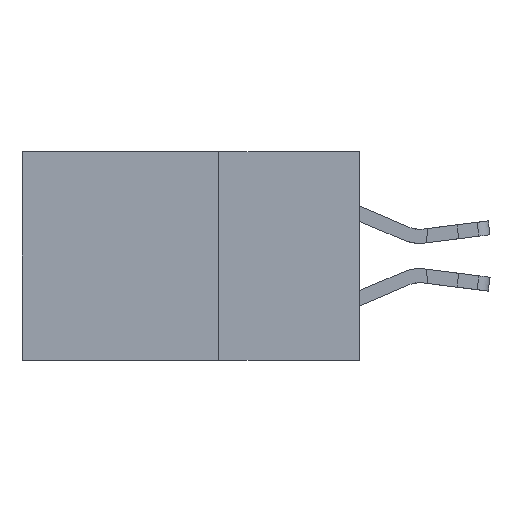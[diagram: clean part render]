
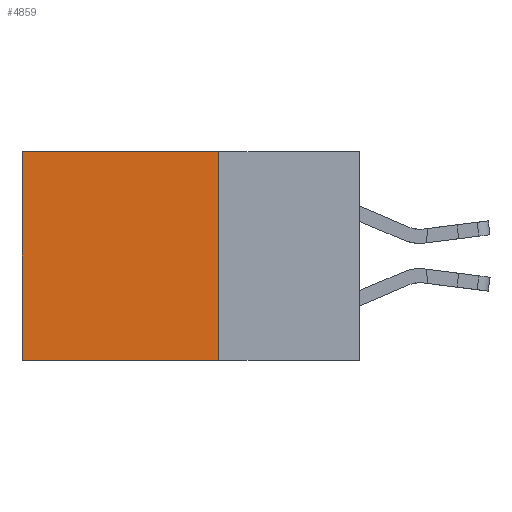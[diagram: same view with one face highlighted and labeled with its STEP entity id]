
A CAD part, left-side view. The second image highlights one B-rep face of the part: STEP entity #4859.
In plain terms, the highlighted planar face has unit normal (-1, 0, 0).
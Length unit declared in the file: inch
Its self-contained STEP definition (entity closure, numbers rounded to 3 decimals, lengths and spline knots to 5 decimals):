
#302 = EDGE_CURVE ( 'NONE', #24637, #29451, #16012, .T. ) ;
#420 = ORIENTED_EDGE ( 'NONE', *, *, #27359, .T. ) ;
#3857 = ORIENTED_EDGE ( 'NONE', *, *, #10901, .T. ) ;
#4203 = VECTOR ( 'NONE', #13015, 39.37008 ) ;
#4370 = DIRECTION ( 'NONE',  ( 0., 0., -1. ) ) ;
#4859 = ADVANCED_FACE ( 'NONE', ( #28854 ), #28910, .F. ) ;
#6079 = ORIENTED_EDGE ( 'NONE', *, *, #302, .F. ) ;
#6340 = ORIENTED_EDGE ( 'NONE', *, *, #11424, .F. ) ;
#8848 = CARTESIAN_POINT ( 'NONE',  ( 0.2875, 0.6, 0. ) ) ;
#9048 = LINE ( 'NONE', #17843, #19041 ) ;
#10865 = DIRECTION ( 'NONE',  ( 1., 0., 0. ) ) ;
#10901 = EDGE_CURVE ( 'NONE', #28396, #12480, #9048, .T. ) ;
#11424 = EDGE_CURVE ( 'NONE', #29451, #12480, #16415, .T. ) ;
#12384 = DIRECTION ( 'NONE',  ( 0., 0., -1. ) ) ;
#12480 = VERTEX_POINT ( 'NONE', #19694 ) ;
#13015 = DIRECTION ( 'NONE',  ( 0., 1., 0. ) ) ;
#13326 = DIRECTION ( 'NONE',  ( 0., 0., -1. ) ) ;
#13767 = CARTESIAN_POINT ( 'NONE',  ( 0.2875, 0.25, 0. ) ) ;
#14793 = CARTESIAN_POINT ( 'NONE',  ( 0.2875, 0.25, 0. ) ) ;
#16012 = LINE ( 'NONE', #16991, #21148 ) ;
#16415 = LINE ( 'NONE', #26955, #4203 ) ;
#16435 = DIRECTION ( 'NONE',  ( 0., 1., 0. ) ) ;
#16652 = CARTESIAN_POINT ( 'NONE',  ( 0.2875, 0.25, 0. ) ) ;
#16991 = CARTESIAN_POINT ( 'NONE',  ( 0.2875, 0.25, 0. ) ) ;
#17044 = CARTESIAN_POINT ( 'NONE',  ( 0.2875, 0.25, -0.37 ) ) ;
#17843 = CARTESIAN_POINT ( 'NONE',  ( 0.2875, 0.6, 0. ) ) ;
#19041 = VECTOR ( 'NONE', #4370, 39.37008 ) ;
#19694 = CARTESIAN_POINT ( 'NONE',  ( 0.2875, 0.6, -0.37 ) ) ;
#21148 = VECTOR ( 'NONE', #13326, 39.37008 ) ;
#21487 = LINE ( 'NONE', #13767, #28457 ) ;
#24583 = EDGE_LOOP ( 'NONE', ( #3857, #6340, #6079, #420 ) ) ;
#24637 = VERTEX_POINT ( 'NONE', #16652 ) ;
#26675 = AXIS2_PLACEMENT_3D ( 'NONE', #14793, #10865, #12384 ) ;
#26955 = CARTESIAN_POINT ( 'NONE',  ( 0.2875, 0.25, -0.37 ) ) ;
#27359 = EDGE_CURVE ( 'NONE', #24637, #28396, #21487, .T. ) ;
#28396 = VERTEX_POINT ( 'NONE', #8848 ) ;
#28457 = VECTOR ( 'NONE', #16435, 39.37008 ) ;
#28854 = FACE_OUTER_BOUND ( 'NONE', #24583, .T. ) ;
#28910 = PLANE ( 'NONE',  #26675 ) ;
#29451 = VERTEX_POINT ( 'NONE', #17044 ) ;
